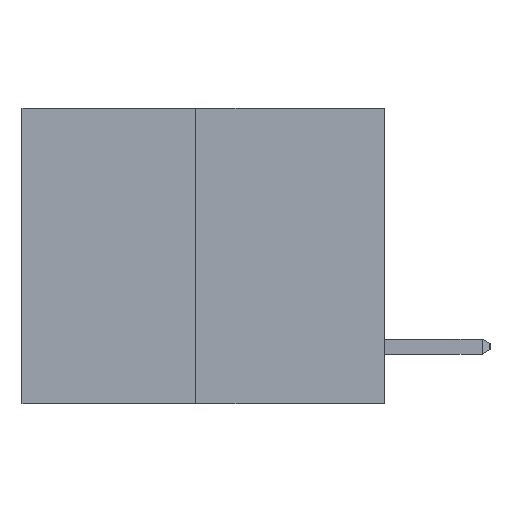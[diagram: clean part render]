
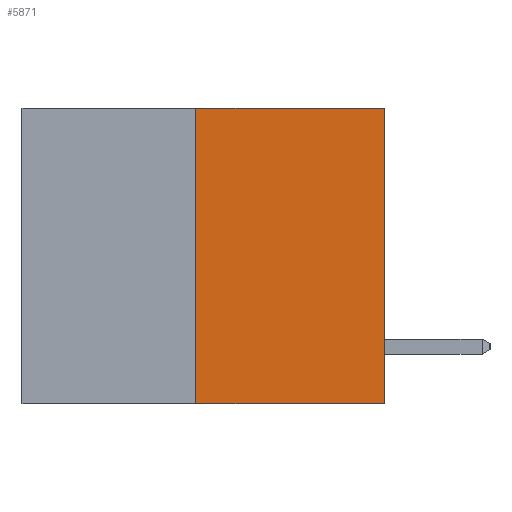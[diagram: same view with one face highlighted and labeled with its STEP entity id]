
A CAD part, left-side view. The second image highlights one B-rep face of the part: STEP entity #5871.
In plain terms, the highlighted planar face has unit normal (-1, 0, 0).
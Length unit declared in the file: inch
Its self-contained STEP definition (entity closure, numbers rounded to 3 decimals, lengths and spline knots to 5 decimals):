
#152 = CARTESIAN_POINT ( 'NONE',  ( 0., 0.312, 0. ) ) ;
#182 = VERTEX_POINT ( 'NONE', #2153 ) ;
#406 = DIRECTION ( 'NONE',  ( 0., 0., 1. ) ) ;
#982 = LINE ( 'NONE', #10805, #14769 ) ;
#1005 = CARTESIAN_POINT ( 'NONE',  ( 0., 0.312, -0.49 ) ) ;
#1302 = DIRECTION ( 'NONE',  ( 1., 0., 0. ) ) ;
#2153 = CARTESIAN_POINT ( 'NONE',  ( 0., 0., 0. ) ) ;
#2341 = PLANE ( 'NONE',  #11478 ) ;
#2915 = DIRECTION ( 'NONE',  ( 0., -1., 0. ) ) ;
#3260 = DIRECTION ( 'NONE',  ( 0., 0., 1. ) ) ;
#3323 = LINE ( 'NONE', #4007, #10913 ) ;
#3490 = EDGE_LOOP ( 'NONE', ( #8948, #12859, #14694, #10087 ) ) ;
#4007 = CARTESIAN_POINT ( 'NONE',  ( 0., 0.6, 0. ) ) ;
#4735 = EDGE_CURVE ( 'NONE', #8656, #182, #3323, .T. ) ;
#4917 = LINE ( 'NONE', #14042, #5982 ) ;
#5407 = EDGE_CURVE ( 'NONE', #12284, #8656, #13493, .T. ) ;
#5871 = ADVANCED_FACE ( 'NONE', ( #8541 ), #2341, .F. ) ;
#5932 = DIRECTION ( 'NONE',  ( 0., 0., -1. ) ) ;
#5982 = VECTOR ( 'NONE', #406, 39.37008 ) ;
#6136 = DIRECTION ( 'NONE',  ( 0., -1., 0. ) ) ;
#7057 = EDGE_CURVE ( 'NONE', #12284, #14500, #982, .T. ) ;
#8213 = CARTESIAN_POINT ( 'NONE',  ( 0., 0.6, 0. ) ) ;
#8541 = FACE_OUTER_BOUND ( 'NONE', #3490, .T. ) ;
#8546 = CARTESIAN_POINT ( 'NONE',  ( 0., 0., -0.49 ) ) ;
#8656 = VERTEX_POINT ( 'NONE', #152 ) ;
#8948 = ORIENTED_EDGE ( 'NONE', *, *, #5407, .F. ) ;
#10087 = ORIENTED_EDGE ( 'NONE', *, *, #4735, .F. ) ;
#10805 = CARTESIAN_POINT ( 'NONE',  ( 0., 0.6, -0.49 ) ) ;
#10913 = VECTOR ( 'NONE', #2915, 39.37008 ) ;
#11478 = AXIS2_PLACEMENT_3D ( 'NONE', #8213, #1302, #5932 ) ;
#12284 = VERTEX_POINT ( 'NONE', #1005 ) ;
#12859 = ORIENTED_EDGE ( 'NONE', *, *, #7057, .T. ) ;
#13493 = LINE ( 'NONE', #14699, #14033 ) ;
#13695 = EDGE_CURVE ( 'NONE', #14500, #182, #4917, .T. ) ;
#14033 = VECTOR ( 'NONE', #3260, 39.37008 ) ;
#14042 = CARTESIAN_POINT ( 'NONE',  ( 0., 0., 0. ) ) ;
#14500 = VERTEX_POINT ( 'NONE', #8546 ) ;
#14694 = ORIENTED_EDGE ( 'NONE', *, *, #13695, .T. ) ;
#14699 = CARTESIAN_POINT ( 'NONE',  ( 0., 0.312, -0.49 ) ) ;
#14769 = VECTOR ( 'NONE', #6136, 39.37008 ) ;
